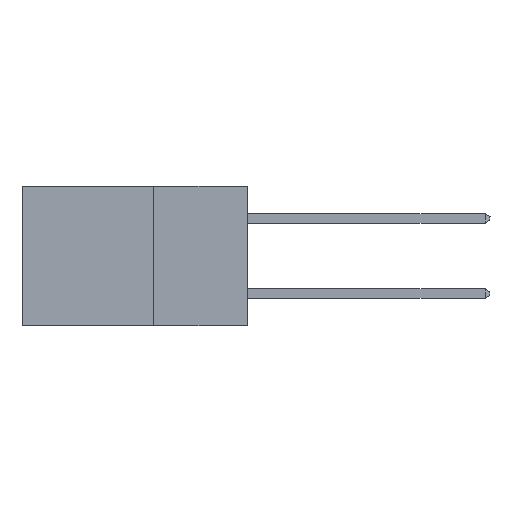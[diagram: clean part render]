
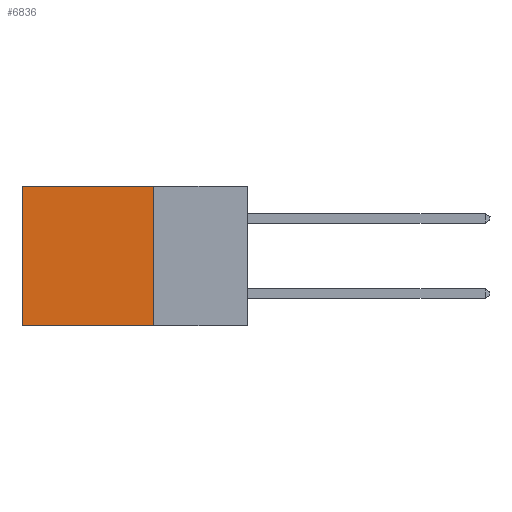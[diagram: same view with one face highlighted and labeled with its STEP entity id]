
A CAD part, left-side view. The second image highlights one B-rep face of the part: STEP entity #6836.
In plain terms, the highlighted planar face has unit normal (-1, 0, 0).
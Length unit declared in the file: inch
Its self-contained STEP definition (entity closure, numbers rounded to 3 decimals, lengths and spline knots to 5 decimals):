
#360 = EDGE_CURVE ( 'NONE', #20461, #17726, #8296, .T. ) ;
#540 = DIRECTION ( 'NONE',  ( 1., 0., 0. ) ) ;
#796 = VECTOR ( 'NONE', #13819, 39.37008 ) ;
#1070 = LINE ( 'NONE', #22942, #13296 ) ;
#1504 = CARTESIAN_POINT ( 'NONE',  ( 0.2615, 0.25, 0. ) ) ;
#2108 = LINE ( 'NONE', #2816, #20802 ) ;
#2816 = CARTESIAN_POINT ( 'NONE',  ( 0.2615, 0.25, 0. ) ) ;
#4718 = ORIENTED_EDGE ( 'NONE', *, *, #360, .F. ) ;
#4730 = CARTESIAN_POINT ( 'NONE',  ( 0.2615, 0.25, -0.37 ) ) ;
#5307 = CARTESIAN_POINT ( 'NONE',  ( 0.2615, 0.6, -0.37 ) ) ;
#6119 = VERTEX_POINT ( 'NONE', #10879 ) ;
#6508 = CARTESIAN_POINT ( 'NONE',  ( 0.2615, 0.25, -0.37 ) ) ;
#6524 = PLANE ( 'NONE',  #12040 ) ;
#6605 = ORIENTED_EDGE ( 'NONE', *, *, #13339, .T. ) ;
#6836 = ADVANCED_FACE ( 'NONE', ( #9755 ), #6524, .F. ) ;
#7840 = DIRECTION ( 'NONE',  ( 0., 0., -1. ) ) ;
#8296 = LINE ( 'NONE', #6508, #16453 ) ;
#9055 = VERTEX_POINT ( 'NONE', #18437 ) ;
#9586 = EDGE_CURVE ( 'NONE', #17726, #6119, #1070, .T. ) ;
#9755 = FACE_OUTER_BOUND ( 'NONE', #16175, .T. ) ;
#10794 = LINE ( 'NONE', #5307, #796 ) ;
#10879 = CARTESIAN_POINT ( 'NONE',  ( 0.2615, 0.6, -0.37 ) ) ;
#11560 = DIRECTION ( 'NONE',  ( 0., 1., 0. ) ) ;
#11605 = CARTESIAN_POINT ( 'NONE',  ( 0.2615, 0.25, -0.37 ) ) ;
#12040 = AXIS2_PLACEMENT_3D ( 'NONE', #4730, #540, #7840 ) ;
#13296 = VECTOR ( 'NONE', #15173, 39.37008 ) ;
#13339 = EDGE_CURVE ( 'NONE', #9055, #6119, #10794, .T. ) ;
#13802 = DIRECTION ( 'NONE',  ( 0., 0., -1. ) ) ;
#13819 = DIRECTION ( 'NONE',  ( 0., 0., -1. ) ) ;
#15173 = DIRECTION ( 'NONE',  ( 0., 1., 0. ) ) ;
#16175 = EDGE_LOOP ( 'NONE', ( #6605, #16777, #4718, #20598 ) ) ;
#16453 = VECTOR ( 'NONE', #13802, 39.37008 ) ;
#16777 = ORIENTED_EDGE ( 'NONE', *, *, #9586, .F. ) ;
#17726 = VERTEX_POINT ( 'NONE', #11605 ) ;
#18437 = CARTESIAN_POINT ( 'NONE',  ( 0.2615, 0.6, 0. ) ) ;
#20461 = VERTEX_POINT ( 'NONE', #1504 ) ;
#20598 = ORIENTED_EDGE ( 'NONE', *, *, #21618, .T. ) ;
#20802 = VECTOR ( 'NONE', #11560, 39.37008 ) ;
#21618 = EDGE_CURVE ( 'NONE', #20461, #9055, #2108, .T. ) ;
#22942 = CARTESIAN_POINT ( 'NONE',  ( 0.2615, 0.25, -0.37 ) ) ;
